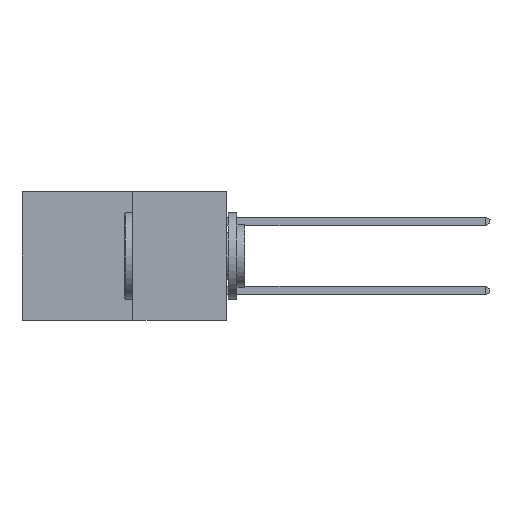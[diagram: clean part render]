
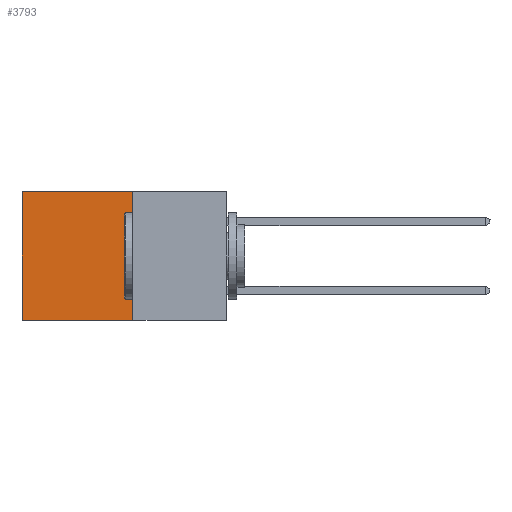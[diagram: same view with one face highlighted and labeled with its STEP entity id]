
A CAD part, left-side view. The second image highlights one B-rep face of the part: STEP entity #3793.
In plain terms, the highlighted planar face has unit normal (-1, 0, 0).
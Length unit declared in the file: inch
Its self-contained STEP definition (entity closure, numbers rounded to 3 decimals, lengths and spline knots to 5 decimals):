
#25 = DIRECTION ( 'NONE',  ( 0., 1., 0. ) ) ;
#153 = VECTOR ( 'NONE', #2868, 39.37008 ) ;
#381 = VECTOR ( 'NONE', #7516, 39.37008 ) ;
#471 = LINE ( 'NONE', #7337, #7309 ) ;
#729 = ORIENTED_EDGE ( 'NONE', *, *, #2516, .T. ) ;
#759 = CARTESIAN_POINT ( 'NONE',  ( 0.277, 0.59, -0.37 ) ) ;
#1200 = VERTEX_POINT ( 'NONE', #6335 ) ;
#1891 = CARTESIAN_POINT ( 'NONE',  ( 0.277, 0.27, -0.37 ) ) ;
#1933 = ORIENTED_EDGE ( 'NONE', *, *, #8180, .T. ) ;
#1945 = VECTOR ( 'NONE', #25, 39.37008 ) ;
#2166 = LINE ( 'NONE', #5014, #381 ) ;
#2277 = EDGE_CURVE ( 'NONE', #3125, #3404, #471, .T. ) ;
#2516 = EDGE_CURVE ( 'NONE', #7530, #3404, #5338, .T. ) ;
#2868 = DIRECTION ( 'NONE',  ( 0., 0., -1. ) ) ;
#3125 = VERTEX_POINT ( 'NONE', #1891 ) ;
#3397 = ORIENTED_EDGE ( 'NONE', *, *, #2277, .F. ) ;
#3404 = VERTEX_POINT ( 'NONE', #759 ) ;
#3406 = DIRECTION ( 'NONE',  ( 1., 0., 0. ) ) ;
#3467 = AXIS2_PLACEMENT_3D ( 'NONE', #6003, #3406, #6361 ) ;
#3661 = ORIENTED_EDGE ( 'NONE', *, *, #7233, .F. ) ;
#3793 = ADVANCED_FACE ( 'NONE', ( #8170 ), #6845, .F. ) ;
#5014 = CARTESIAN_POINT ( 'NONE',  ( 0.277, 0.27, -0.37 ) ) ;
#5338 = LINE ( 'NONE', #5601, #153 ) ;
#5348 = EDGE_LOOP ( 'NONE', ( #729, #3397, #3661, #1933 ) ) ;
#5536 = LINE ( 'NONE', #7752, #1945 ) ;
#5601 = CARTESIAN_POINT ( 'NONE',  ( 0.277, 0.59, -0.37 ) ) ;
#5904 = CARTESIAN_POINT ( 'NONE',  ( 0.277, 0.59, 0. ) ) ;
#6003 = CARTESIAN_POINT ( 'NONE',  ( 0.277, 0.27, -0.37 ) ) ;
#6335 = CARTESIAN_POINT ( 'NONE',  ( 0.277, 0.27, 0. ) ) ;
#6361 = DIRECTION ( 'NONE',  ( 0., 0., -1. ) ) ;
#6845 = PLANE ( 'NONE',  #3467 ) ;
#7233 = EDGE_CURVE ( 'NONE', #1200, #3125, #2166, .T. ) ;
#7308 = DIRECTION ( 'NONE',  ( 0., 1., 0. ) ) ;
#7309 = VECTOR ( 'NONE', #7308, 39.37008 ) ;
#7337 = CARTESIAN_POINT ( 'NONE',  ( 0.277, 0.27, -0.37 ) ) ;
#7516 = DIRECTION ( 'NONE',  ( 0., 0., -1. ) ) ;
#7530 = VERTEX_POINT ( 'NONE', #5904 ) ;
#7752 = CARTESIAN_POINT ( 'NONE',  ( 0.277, 0.27, 0. ) ) ;
#8170 = FACE_OUTER_BOUND ( 'NONE', #5348, .T. ) ;
#8180 = EDGE_CURVE ( 'NONE', #1200, #7530, #5536, .T. ) ;
